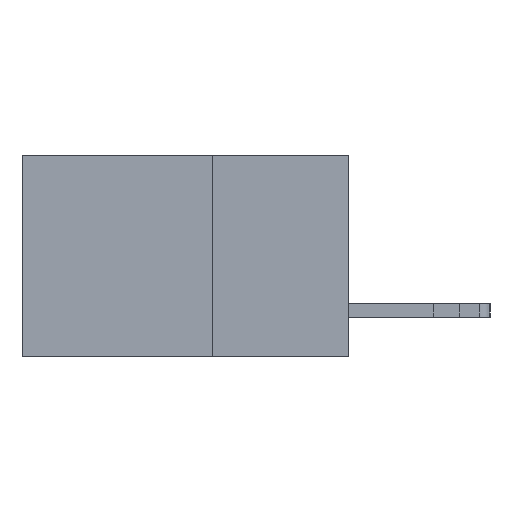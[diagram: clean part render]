
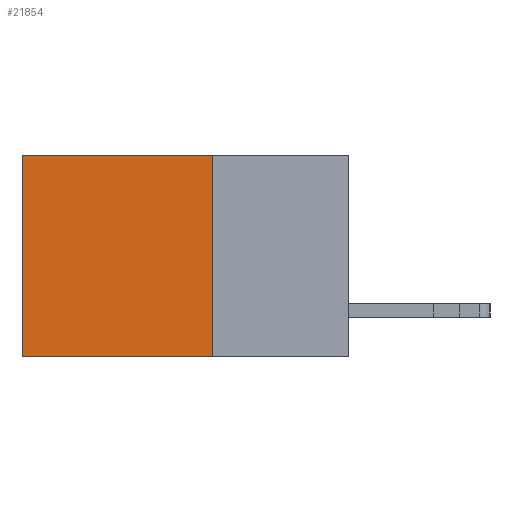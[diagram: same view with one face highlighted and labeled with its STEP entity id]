
A CAD part, left-side view. The second image highlights one B-rep face of the part: STEP entity #21854.
In plain terms, the highlighted planar face has unit normal (-1, 0, 0).
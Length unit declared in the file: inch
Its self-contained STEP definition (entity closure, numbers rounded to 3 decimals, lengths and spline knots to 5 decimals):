
#343 = LINE ( 'NONE', #12469, #18824 ) ;
#614 = ORIENTED_EDGE ( 'NONE', *, *, #12285, .T. ) ;
#1283 = LINE ( 'NONE', #9203, #10102 ) ;
#1995 = EDGE_CURVE ( 'NONE', #13651, #11178, #1283, .T. ) ;
#2690 = ORIENTED_EDGE ( 'NONE', *, *, #11092, .T. ) ;
#3215 = CARTESIAN_POINT ( 'NONE',  ( 0.298, 0.25, 0. ) ) ;
#4066 = VECTOR ( 'NONE', #7674, 39.37008 ) ;
#4952 = FACE_OUTER_BOUND ( 'NONE', #19762, .T. ) ;
#5718 = LINE ( 'NONE', #5963, #4066 ) ;
#5963 = CARTESIAN_POINT ( 'NONE',  ( 0.298, 0.25, 0. ) ) ;
#6723 = CARTESIAN_POINT ( 'NONE',  ( 0.298, 0.6, 0. ) ) ;
#6743 = AXIS2_PLACEMENT_3D ( 'NONE', #3215, #19318, #8467 ) ;
#7034 = CARTESIAN_POINT ( 'NONE',  ( 0.298, 0.25, -0.37 ) ) ;
#7151 = DIRECTION ( 'NONE',  ( 0., 1., 0. ) ) ;
#7195 = LINE ( 'NONE', #6723, #21005 ) ;
#7301 = CARTESIAN_POINT ( 'NONE',  ( 0.298, 0.6, -0.37 ) ) ;
#7674 = DIRECTION ( 'NONE',  ( 0., 0., -1. ) ) ;
#8467 = DIRECTION ( 'NONE',  ( 0., 0., -1. ) ) ;
#8482 = DIRECTION ( 'NONE',  ( 0., 0., -1. ) ) ;
#9203 = CARTESIAN_POINT ( 'NONE',  ( 0.298, 0.25, -0.37 ) ) ;
#9212 = VERTEX_POINT ( 'NONE', #17129 ) ;
#10102 = VECTOR ( 'NONE', #18493, 39.37008 ) ;
#11092 = EDGE_CURVE ( 'NONE', #9212, #19887, #343, .T. ) ;
#11178 = VERTEX_POINT ( 'NONE', #7301 ) ;
#12285 = EDGE_CURVE ( 'NONE', #19887, #11178, #7195, .T. ) ;
#12469 = CARTESIAN_POINT ( 'NONE',  ( 0.298, 0.25, 0. ) ) ;
#13651 = VERTEX_POINT ( 'NONE', #7034 ) ;
#15048 = ORIENTED_EDGE ( 'NONE', *, *, #16289, .F. ) ;
#16289 = EDGE_CURVE ( 'NONE', #9212, #13651, #5718, .T. ) ;
#17129 = CARTESIAN_POINT ( 'NONE',  ( 0.298, 0.25, 0. ) ) ;
#17213 = CARTESIAN_POINT ( 'NONE',  ( 0.298, 0.6, 0. ) ) ;
#17539 = PLANE ( 'NONE',  #6743 ) ;
#18493 = DIRECTION ( 'NONE',  ( 0., 1., 0. ) ) ;
#18824 = VECTOR ( 'NONE', #7151, 39.37008 ) ;
#19318 = DIRECTION ( 'NONE',  ( 1., 0., 0. ) ) ;
#19762 = EDGE_LOOP ( 'NONE', ( #614, #21458, #15048, #2690 ) ) ;
#19887 = VERTEX_POINT ( 'NONE', #17213 ) ;
#21005 = VECTOR ( 'NONE', #8482, 39.37008 ) ;
#21458 = ORIENTED_EDGE ( 'NONE', *, *, #1995, .F. ) ;
#21854 = ADVANCED_FACE ( 'NONE', ( #4952 ), #17539, .F. ) ;
